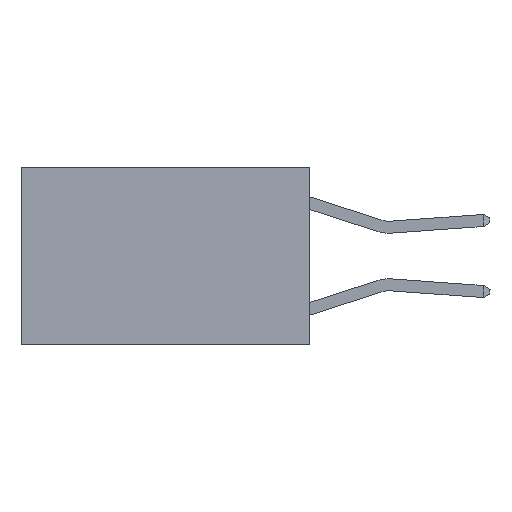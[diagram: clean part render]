
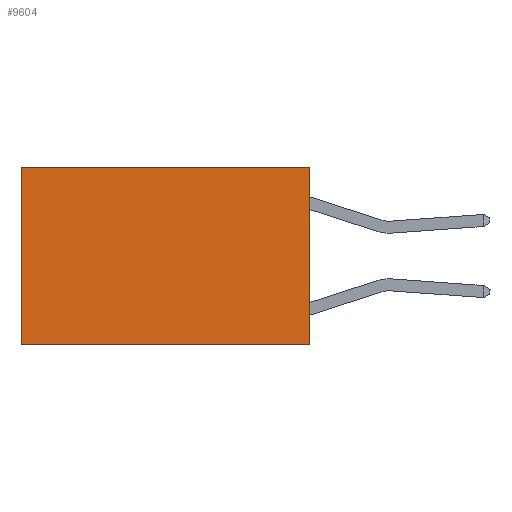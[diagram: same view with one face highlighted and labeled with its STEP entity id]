
A CAD part, left-side view. The second image highlights one B-rep face of the part: STEP entity #9604.
In plain terms, the highlighted planar face has unit normal (-1, 0, 0).
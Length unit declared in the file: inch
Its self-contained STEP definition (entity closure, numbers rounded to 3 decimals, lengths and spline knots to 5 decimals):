
#163 = EDGE_LOOP ( 'NONE', ( #12971, #7960, #5666, #9616 ) ) ;
#186 = VERTEX_POINT ( 'NONE', #2698 ) ;
#388 = LINE ( 'NONE', #6985, #12598 ) ;
#1583 = EDGE_CURVE ( 'NONE', #3187, #1742, #7150, .T. ) ;
#1736 = EDGE_CURVE ( 'NONE', #186, #3232, #12370, .T. ) ;
#1742 = VERTEX_POINT ( 'NONE', #12537 ) ;
#1814 = PLANE ( 'NONE',  #5355 ) ;
#2698 = CARTESIAN_POINT ( 'NONE',  ( 0.2625, 0., 0. ) ) ;
#3133 = DIRECTION ( 'NONE',  ( 0., 1., 0. ) ) ;
#3168 = VECTOR ( 'NONE', #13333, 39.37008 ) ;
#3187 = VERTEX_POINT ( 'NONE', #13925 ) ;
#3207 = DIRECTION ( 'NONE',  ( 0., 0., -1. ) ) ;
#3232 = VERTEX_POINT ( 'NONE', #9208 ) ;
#3648 = EDGE_CURVE ( 'NONE', #3232, #1742, #5000, .T. ) ;
#5000 = LINE ( 'NONE', #10199, #12835 ) ;
#5355 = AXIS2_PLACEMENT_3D ( 'NONE', #7288, #12260, #5840 ) ;
#5666 = ORIENTED_EDGE ( 'NONE', *, *, #12265, .F. ) ;
#5753 = FACE_OUTER_BOUND ( 'NONE', #163, .T. ) ;
#5840 = DIRECTION ( 'NONE',  ( 0., 0., -1. ) ) ;
#6466 = VECTOR ( 'NONE', #3133, 39.37008 ) ;
#6985 = CARTESIAN_POINT ( 'NONE',  ( 0.2625, 0., 0. ) ) ;
#7069 = CARTESIAN_POINT ( 'NONE',  ( 0.2625, 0., -0.37 ) ) ;
#7150 = LINE ( 'NONE', #7069, #3168 ) ;
#7288 = CARTESIAN_POINT ( 'NONE',  ( 0.2625, 0., 0. ) ) ;
#7960 = ORIENTED_EDGE ( 'NONE', *, *, #1583, .F. ) ;
#9208 = CARTESIAN_POINT ( 'NONE',  ( 0.2625, 0.6, 0. ) ) ;
#9604 = ADVANCED_FACE ( 'NONE', ( #5753 ), #1814, .F. ) ;
#9616 = ORIENTED_EDGE ( 'NONE', *, *, #1736, .T. ) ;
#9641 = CARTESIAN_POINT ( 'NONE',  ( 0.2625, 0., 0. ) ) ;
#10199 = CARTESIAN_POINT ( 'NONE',  ( 0.2625, 0.6, 0. ) ) ;
#12260 = DIRECTION ( 'NONE',  ( 1., 0., 0. ) ) ;
#12265 = EDGE_CURVE ( 'NONE', #186, #3187, #388, .T. ) ;
#12370 = LINE ( 'NONE', #9641, #6466 ) ;
#12537 = CARTESIAN_POINT ( 'NONE',  ( 0.2625, 0.6, -0.37 ) ) ;
#12598 = VECTOR ( 'NONE', #3207, 39.37008 ) ;
#12835 = VECTOR ( 'NONE', #15447, 39.37008 ) ;
#12971 = ORIENTED_EDGE ( 'NONE', *, *, #3648, .T. ) ;
#13333 = DIRECTION ( 'NONE',  ( 0., 1., 0. ) ) ;
#13925 = CARTESIAN_POINT ( 'NONE',  ( 0.2625, 0., -0.37 ) ) ;
#15447 = DIRECTION ( 'NONE',  ( 0., 0., -1. ) ) ;
